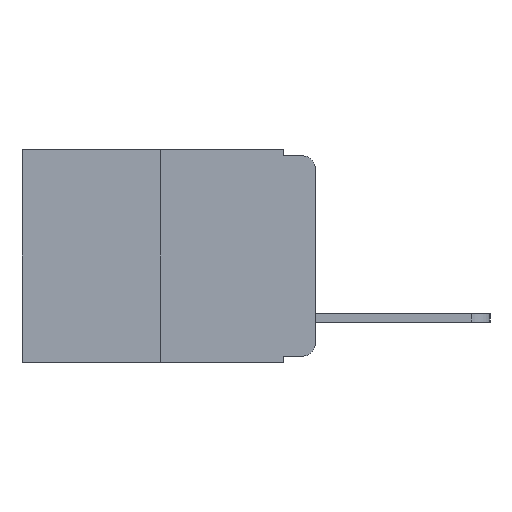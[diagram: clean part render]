
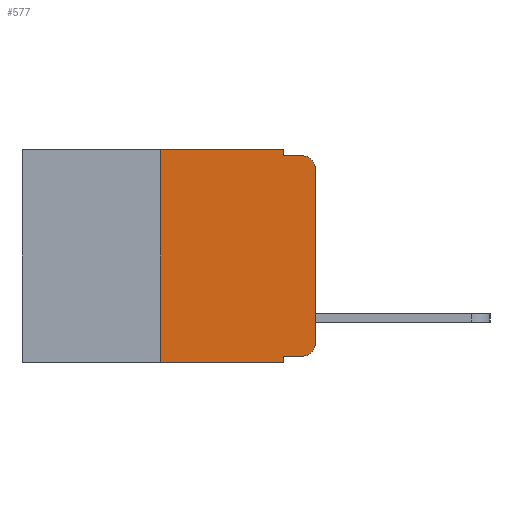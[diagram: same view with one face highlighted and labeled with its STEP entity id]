
A CAD part, left-side view. The second image highlights one B-rep face of the part: STEP entity #577.
In plain terms, the highlighted planar face has unit normal (-1, 0, 0).
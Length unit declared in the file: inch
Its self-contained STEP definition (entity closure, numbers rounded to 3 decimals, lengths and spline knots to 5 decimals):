
#253 = CARTESIAN_POINT ( 'NONE',  ( 0., 0.051, -0.333 ) ) ;
#577 = ADVANCED_FACE ( 'NONE', ( #4742 ), #2745, .F. ) ;
#756 = ORIENTED_EDGE ( 'NONE', *, *, #3076, .F. ) ;
#910 = EDGE_CURVE ( 'NONE', #5797, #12045, #1074, .T. ) ;
#912 = CARTESIAN_POINT ( 'NONE',  ( 0., 0.473, 0. ) ) ;
#1074 = LINE ( 'NONE', #3802, #12292 ) ;
#1165 = EDGE_CURVE ( 'NONE', #4860, #5797, #6698, .T. ) ;
#1267 = DIRECTION ( 'NONE',  ( -1., 0., 0. ) ) ;
#1438 = CARTESIAN_POINT ( 'NONE',  ( 0., 0.051, -0.01 ) ) ;
#2071 = AXIS2_PLACEMENT_3D ( 'NONE', #5830, #13417, #6930 ) ;
#2160 = DIRECTION ( 'NONE',  ( 0., 0., -1. ) ) ;
#2161 = CARTESIAN_POINT ( 'NONE',  ( 0., 0.02, -0.333 ) ) ;
#2192 = CARTESIAN_POINT ( 'NONE',  ( 0., 0.051, 0. ) ) ;
#2621 = CIRCLE ( 'NONE', #12518, 0.02 ) ;
#2723 = LINE ( 'NONE', #5394, #13974 ) ;
#2745 = PLANE ( 'NONE',  #7921 ) ;
#2830 = DIRECTION ( 'NONE',  ( 1., 0., 0. ) ) ;
#2868 = CARTESIAN_POINT ( 'NONE',  ( 0., 0.051, -0.343 ) ) ;
#2869 = DIRECTION ( 'NONE',  ( 0., 0., -1. ) ) ;
#3076 = EDGE_CURVE ( 'NONE', #3524, #7910, #13676, .T. ) ;
#3290 = VERTEX_POINT ( 'NONE', #13082 ) ;
#3512 = DIRECTION ( 'NONE',  ( 0., -1., 0. ) ) ;
#3520 = EDGE_CURVE ( 'NONE', #3290, #5912, #10407, .T. ) ;
#3524 = VERTEX_POINT ( 'NONE', #5500 ) ;
#3784 = VECTOR ( 'NONE', #10876, 39.37008 ) ;
#3802 = CARTESIAN_POINT ( 'NONE',  ( 0., 0.473, 0. ) ) ;
#4332 = CARTESIAN_POINT ( 'NONE',  ( 0., 0.051, -0.333 ) ) ;
#4392 = ORIENTED_EDGE ( 'NONE', *, *, #7471, .T. ) ;
#4482 = VECTOR ( 'NONE', #3512, 39.37008 ) ;
#4742 = FACE_OUTER_BOUND ( 'NONE', #11245, .T. ) ;
#4860 = VERTEX_POINT ( 'NONE', #10533 ) ;
#4980 = VECTOR ( 'NONE', #6483, 39.37008 ) ;
#5201 = ORIENTED_EDGE ( 'NONE', *, *, #9169, .F. ) ;
#5281 = CARTESIAN_POINT ( 'NONE',  ( 0., 0.02, -0.01 ) ) ;
#5394 = CARTESIAN_POINT ( 'NONE',  ( 0., 0.051, 0. ) ) ;
#5500 = CARTESIAN_POINT ( 'NONE',  ( 0., 0.051, -0.01 ) ) ;
#5604 = ORIENTED_EDGE ( 'NONE', *, *, #3520, .T. ) ;
#5797 = VERTEX_POINT ( 'NONE', #11080 ) ;
#5830 = CARTESIAN_POINT ( 'NONE',  ( 0., 0.02, -0.313 ) ) ;
#5910 = ORIENTED_EDGE ( 'NONE', *, *, #7559, .T. ) ;
#5912 = VERTEX_POINT ( 'NONE', #13196 ) ;
#6085 = ORIENTED_EDGE ( 'NONE', *, *, #7534, .T. ) ;
#6206 = CARTESIAN_POINT ( 'NONE',  ( 0., 0.25, 0. ) ) ;
#6235 = DIRECTION ( 'NONE',  ( 0., 0., 1. ) ) ;
#6411 = ORIENTED_EDGE ( 'NONE', *, *, #910, .F. ) ;
#6483 = DIRECTION ( 'NONE',  ( 0., -1., 0. ) ) ;
#6698 = LINE ( 'NONE', #6206, #12110 ) ;
#6713 = LINE ( 'NONE', #2192, #3784 ) ;
#6725 = CIRCLE ( 'NONE', #2071, 0.02 ) ;
#6930 = DIRECTION ( 'NONE',  ( 0., 0., -1. ) ) ;
#7209 = VECTOR ( 'NONE', #10976, 39.37008 ) ;
#7402 = VERTEX_POINT ( 'NONE', #4332 ) ;
#7471 = EDGE_CURVE ( 'NONE', #5912, #7910, #2621, .T. ) ;
#7478 = DIRECTION ( 'NONE',  ( 0., -1., 0. ) ) ;
#7534 = EDGE_CURVE ( 'NONE', #4860, #8999, #13518, .T. ) ;
#7559 = EDGE_CURVE ( 'NONE', #7402, #10294, #13168, .T. ) ;
#7591 = EDGE_CURVE ( 'NONE', #10294, #3290, #6725, .T. ) ;
#7802 = CARTESIAN_POINT ( 'NONE',  ( 0., 0.02, -0.03 ) ) ;
#7910 = VERTEX_POINT ( 'NONE', #5281 ) ;
#7921 = AXIS2_PLACEMENT_3D ( 'NONE', #912, #2830, #2869 ) ;
#8008 = EDGE_CURVE ( 'NONE', #7402, #8999, #6713, .T. ) ;
#8859 = DIRECTION ( 'NONE',  ( 0., 0., -1. ) ) ;
#8956 = ORIENTED_EDGE ( 'NONE', *, *, #8008, .F. ) ;
#8996 = DIRECTION ( 'NONE',  ( 0., -1., 0. ) ) ;
#8999 = VERTEX_POINT ( 'NONE', #2868 ) ;
#9169 = EDGE_CURVE ( 'NONE', #12045, #3524, #2723, .T. ) ;
#10030 = CARTESIAN_POINT ( 'NONE',  ( 0., 0.473, -0.343 ) ) ;
#10294 = VERTEX_POINT ( 'NONE', #2161 ) ;
#10407 = LINE ( 'NONE', #10851, #7209 ) ;
#10533 = CARTESIAN_POINT ( 'NONE',  ( 0., 0.25, -0.343 ) ) ;
#10851 = CARTESIAN_POINT ( 'NONE',  ( 0., 0., 0. ) ) ;
#10876 = DIRECTION ( 'NONE',  ( 0., 0., -1. ) ) ;
#10976 = DIRECTION ( 'NONE',  ( 0., 0., 1. ) ) ;
#10991 = ORIENTED_EDGE ( 'NONE', *, *, #7591, .T. ) ;
#11080 = CARTESIAN_POINT ( 'NONE',  ( 0., 0.25, 0. ) ) ;
#11245 = EDGE_LOOP ( 'NONE', ( #5604, #4392, #756, #5201, #6411, #11663, #6085, #8956, #5910, #10991 ) ) ;
#11663 = ORIENTED_EDGE ( 'NONE', *, *, #1165, .F. ) ;
#12045 = VERTEX_POINT ( 'NONE', #14098 ) ;
#12110 = VECTOR ( 'NONE', #6235, 39.37008 ) ;
#12292 = VECTOR ( 'NONE', #7478, 39.37008 ) ;
#12518 = AXIS2_PLACEMENT_3D ( 'NONE', #7802, #1267, #8859 ) ;
#12812 = VECTOR ( 'NONE', #8996, 39.37008 ) ;
#13082 = CARTESIAN_POINT ( 'NONE',  ( 0., 0., -0.313 ) ) ;
#13168 = LINE ( 'NONE', #253, #12812 ) ;
#13196 = CARTESIAN_POINT ( 'NONE',  ( 0., 0., -0.03 ) ) ;
#13417 = DIRECTION ( 'NONE',  ( -1., 0., 0. ) ) ;
#13518 = LINE ( 'NONE', #10030, #4482 ) ;
#13676 = LINE ( 'NONE', #1438, #4980 ) ;
#13974 = VECTOR ( 'NONE', #2160, 39.37008 ) ;
#14098 = CARTESIAN_POINT ( 'NONE',  ( 0., 0.051, 0. ) ) ;
